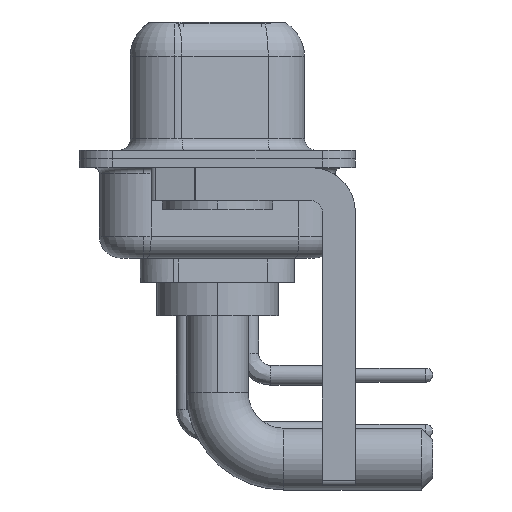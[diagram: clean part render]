
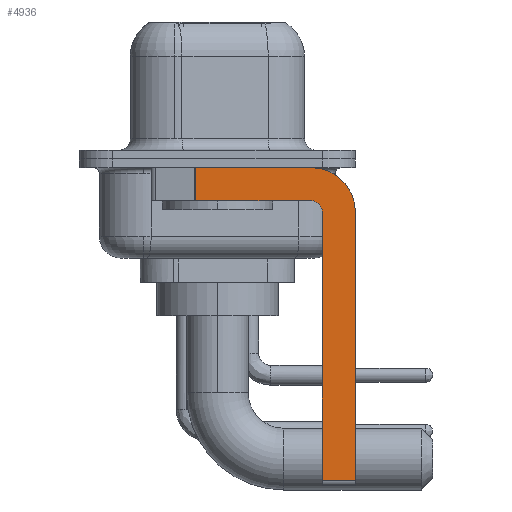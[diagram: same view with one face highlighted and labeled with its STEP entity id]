
A CAD part, left-side view. The second image highlights one B-rep face of the part: STEP entity #4936.
In plain terms, the highlighted planar face has unit normal (-1, 0, 0).
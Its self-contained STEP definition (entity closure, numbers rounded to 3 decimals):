
#528 = ORIENTED_EDGE ( 'NONE', *, *, #3064, .F. ) ;
#810 = LINE ( 'NONE', #12612, #9740 ) ;
#1111 = DIRECTION ( 'NONE',  ( 0., 1., 0. ) ) ;
#1848 = CIRCLE ( 'NONE', #8872, 2. ) ;
#2096 = DIRECTION ( 'NONE',  ( 0., 0., -1. ) ) ;
#2656 = DIRECTION ( 'NONE',  ( 0., 0., 1. ) ) ;
#2699 = CARTESIAN_POINT ( 'NONE',  ( -2.9, 3., -0.4 ) ) ;
#2860 = CARTESIAN_POINT ( 'NONE',  ( -2.9, -4.25, -1.9 ) ) ;
#2945 = VERTEX_POINT ( 'NONE', #20920 ) ;
#3064 = EDGE_CURVE ( 'NONE', #10451, #8402, #9267, .T. ) ;
#3535 = CARTESIAN_POINT ( 'NONE',  ( -2.9, -6.25, -2.4 ) ) ;
#4128 = DIRECTION ( 'NONE',  ( 0., -1., 0. ) ) ;
#4620 = VERTEX_POINT ( 'NONE', #15349 ) ;
#4875 = ORIENTED_EDGE ( 'NONE', *, *, #15413, .T. ) ;
#4936 = ADVANCED_FACE ( 'NONE', ( #20683 ), #10316, .F. ) ;
#5042 = DIRECTION ( 'NONE',  ( 0., 0., 1. ) ) ;
#5128 = DIRECTION ( 'NONE',  ( 0., 0., -1. ) ) ;
#5418 = AXIS2_PLACEMENT_3D ( 'NONE', #14565, #21243, #5042 ) ;
#5936 = AXIS2_PLACEMENT_3D ( 'NONE', #17083, #13688, #2096 ) ;
#6044 = LINE ( 'NONE', #12603, #14793 ) ;
#6594 = ORIENTED_EDGE ( 'NONE', *, *, #9970, .T. ) ;
#6794 = CARTESIAN_POINT ( 'NONE',  ( -2.9, -4.25, -1.9 ) ) ;
#7102 = CARTESIAN_POINT ( 'NONE',  ( -2.9, -4.75, -2.4 ) ) ;
#7857 = CARTESIAN_POINT ( 'NONE',  ( -2.9, 0.978, -1.9 ) ) ;
#7975 = CARTESIAN_POINT ( 'NONE',  ( -2.9, -6.25, -2.4 ) ) ;
#8255 = EDGE_CURVE ( 'NONE', #8402, #13186, #21234, .T. ) ;
#8402 = VERTEX_POINT ( 'NONE', #6794 ) ;
#8501 = VERTEX_POINT ( 'NONE', #17282 ) ;
#8540 = ORIENTED_EDGE ( 'NONE', *, *, #9651, .F. ) ;
#8872 = AXIS2_PLACEMENT_3D ( 'NONE', #9952, #13329, #5128 ) ;
#9133 = EDGE_CURVE ( 'NONE', #2945, #8501, #17370, .T. ) ;
#9267 = CIRCLE ( 'NONE', #5418, 0.5 ) ;
#9651 = EDGE_CURVE ( 'NONE', #4620, #10451, #6044, .T. ) ;
#9740 = VECTOR ( 'NONE', #12506, 1000. ) ;
#9952 = CARTESIAN_POINT ( 'NONE',  ( -2.9, -4.25, -2.4 ) ) ;
#9970 = EDGE_CURVE ( 'NONE', #4620, #18481, #12364, .T. ) ;
#10006 = CARTESIAN_POINT ( 'NONE',  ( -2.9, -6.25, -14.55 ) ) ;
#10122 = ORIENTED_EDGE ( 'NONE', *, *, #9133, .F. ) ;
#10316 = PLANE ( 'NONE',  #5936 ) ;
#10451 = VERTEX_POINT ( 'NONE', #7102 ) ;
#11334 = EDGE_CURVE ( 'NONE', #16458, #18481, #18616, .T. ) ;
#11715 = VECTOR ( 'NONE', #20156, 1000. ) ;
#11894 = ORIENTED_EDGE ( 'NONE', *, *, #20901, .F. ) ;
#12036 = CARTESIAN_POINT ( 'NONE',  ( -2.9, -4.25, -14.55 ) ) ;
#12364 = LINE ( 'NONE', #12036, #16201 ) ;
#12506 = DIRECTION ( 'NONE',  ( 0., 0., -1. ) ) ;
#12603 = CARTESIAN_POINT ( 'NONE',  ( -2.9, -4.75, -14.8 ) ) ;
#12612 = CARTESIAN_POINT ( 'NONE',  ( -2.9, 0.978, -1.9 ) ) ;
#13186 = VERTEX_POINT ( 'NONE', #7857 ) ;
#13329 = DIRECTION ( 'NONE',  ( 1., 0., 0. ) ) ;
#13688 = DIRECTION ( 'NONE',  ( 1., 0., 0. ) ) ;
#14565 = CARTESIAN_POINT ( 'NONE',  ( -2.9, -4.25, -2.4 ) ) ;
#14793 = VECTOR ( 'NONE', #2656, 1000. ) ;
#15349 = CARTESIAN_POINT ( 'NONE',  ( -2.9, -4.75, -14.55 ) ) ;
#15413 = EDGE_CURVE ( 'NONE', #2945, #13186, #810, .T. ) ;
#15676 = VECTOR ( 'NONE', #4128, 1000. ) ;
#16201 = VECTOR ( 'NONE', #17071, 1000. ) ;
#16458 = VERTEX_POINT ( 'NONE', #7975 ) ;
#16555 = VECTOR ( 'NONE', #1111, 1000. ) ;
#17071 = DIRECTION ( 'NONE',  ( 0., -1., 0. ) ) ;
#17083 = CARTESIAN_POINT ( 'NONE',  ( -2.9, -4.25, -2.4 ) ) ;
#17272 = EDGE_LOOP ( 'NONE', ( #10122, #4875, #18256, #528, #8540, #6594, #18450, #11894 ) ) ;
#17282 = CARTESIAN_POINT ( 'NONE',  ( -2.9, -4.25, -0.4 ) ) ;
#17370 = LINE ( 'NONE', #2699, #15676 ) ;
#18256 = ORIENTED_EDGE ( 'NONE', *, *, #8255, .F. ) ;
#18450 = ORIENTED_EDGE ( 'NONE', *, *, #11334, .F. ) ;
#18481 = VERTEX_POINT ( 'NONE', #10006 ) ;
#18616 = LINE ( 'NONE', #3535, #11715 ) ;
#20156 = DIRECTION ( 'NONE',  ( 0., 0., -1. ) ) ;
#20683 = FACE_OUTER_BOUND ( 'NONE', #17272, .T. ) ;
#20901 = EDGE_CURVE ( 'NONE', #8501, #16458, #1848, .T. ) ;
#20920 = CARTESIAN_POINT ( 'NONE',  ( -2.9, 0.978, -0.4 ) ) ;
#21234 = LINE ( 'NONE', #2860, #16555 ) ;
#21243 = DIRECTION ( 'NONE',  ( -1., 0., 0. ) ) ;
